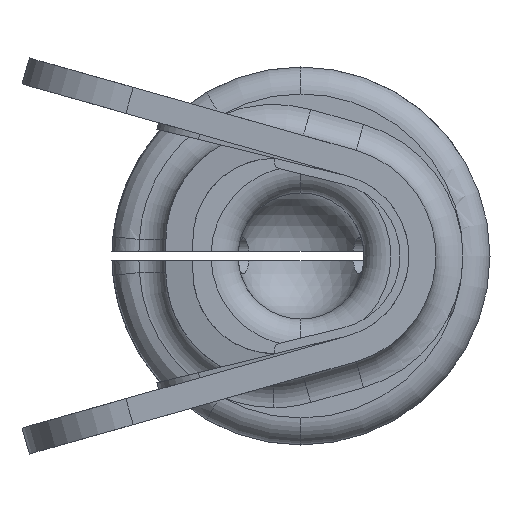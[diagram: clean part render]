
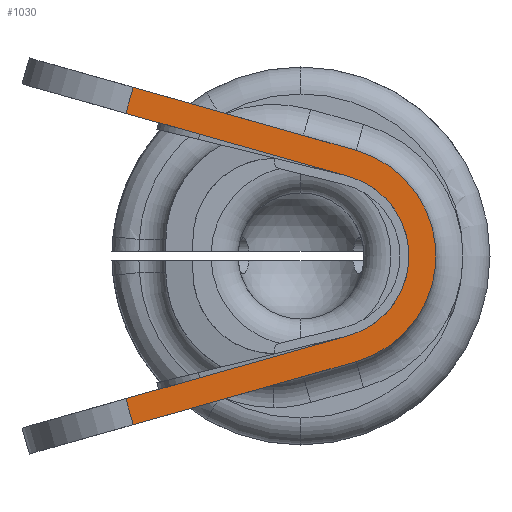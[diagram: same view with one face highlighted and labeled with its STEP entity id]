
A CAD part, left-side view. The second image highlights one B-rep face of the part: STEP entity #1030.
In plain terms, the highlighted planar face has unit normal (-1, 0, 0).
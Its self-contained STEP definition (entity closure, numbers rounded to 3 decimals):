
#196 = ORIENTED_EDGE ( 'NONE', *, *, #3248, .T. ) ;
#217 = CARTESIAN_POINT ( 'NONE',  ( -12.88, -0.106, -0.374 ) ) ;
#218 = VECTOR ( 'NONE', #5639, 1000. ) ;
#318 = ORIENTED_EDGE ( 'NONE', *, *, #1427, .T. ) ;
#349 = CIRCLE ( 'NONE', #6018, 0.46 ) ;
#354 = VECTOR ( 'NONE', #6007, 1000. ) ;
#433 = VECTOR ( 'NONE', #5708, 1000. ) ;
#526 = VERTEX_POINT ( 'NONE', #4530 ) ;
#736 = DIRECTION ( 'NONE',  ( 0., 0., -1. ) ) ;
#853 = CARTESIAN_POINT ( 'NONE',  ( -12.88, 0.26, 0. ) ) ;
#873 = EDGE_LOOP ( 'NONE', ( #5237, #196, #3596, #5016, #2593, #318, #3690, #2170 ) ) ;
#914 = VERTEX_POINT ( 'NONE', #3044 ) ;
#1030 = ADVANCED_FACE ( 'NONE', ( #2239 ), #1643, .F. ) ;
#1034 = CARTESIAN_POINT ( 'NONE',  ( -12.88, -0.147, 0.519 ) ) ;
#1427 = EDGE_CURVE ( 'NONE', #914, #5588, #1929, .T. ) ;
#1455 = CARTESIAN_POINT ( 'NONE',  ( -12.88, 1.332, -0.937 ) ) ;
#1634 = CARTESIAN_POINT ( 'NONE',  ( -12.88, 0.26, 0. ) ) ;
#1643 = PLANE ( 'NONE',  #5161 ) ;
#1670 = LINE ( 'NONE', #3774, #3249 ) ;
#1888 = CARTESIAN_POINT ( 'NONE',  ( -12.88, -0.106, 0.374 ) ) ;
#1929 = LINE ( 'NONE', #1455, #354 ) ;
#2170 = ORIENTED_EDGE ( 'NONE', *, *, #2978, .F. ) ;
#2176 = CIRCLE ( 'NONE', #4102, 0.61 ) ;
#2220 = DIRECTION ( 'NONE',  ( 0., 0.272, -0.962 ) ) ;
#2239 = FACE_OUTER_BOUND ( 'NONE', #873, .T. ) ;
#2341 = VERTEX_POINT ( 'NONE', #6127 ) ;
#2424 = DIRECTION ( 'NONE',  ( 0., -0.962, -0.272 ) ) ;
#2428 = EDGE_CURVE ( 'NONE', #5588, #526, #1670, .T. ) ;
#2438 = EDGE_CURVE ( 'NONE', #5448, #2341, #349, .T. ) ;
#2593 = ORIENTED_EDGE ( 'NONE', *, *, #5847, .F. ) ;
#2687 = CARTESIAN_POINT ( 'NONE',  ( -12.88, 0., 0. ) ) ;
#2916 = DIRECTION ( 'NONE',  ( 1., 0., 0. ) ) ;
#2974 = VERTEX_POINT ( 'NONE', #4367 ) ;
#2978 = EDGE_CURVE ( 'NONE', #6086, #526, #2176, .T. ) ;
#3028 = LINE ( 'NONE', #1034, #218 ) ;
#3044 = CARTESIAN_POINT ( 'NONE',  ( -12.88, 1.373, -0.792 ) ) ;
#3157 = DIRECTION ( 'NONE',  ( 1., 0., 0. ) ) ;
#3213 = DIRECTION ( 'NONE',  ( 0., 0., -1. ) ) ;
#3248 = EDGE_CURVE ( 'NONE', #2974, #4641, #3761, .T. ) ;
#3249 = VECTOR ( 'NONE', #5308, 1000. ) ;
#3487 = CARTESIAN_POINT ( 'NONE',  ( -12.88, 1.332, -0.937 ) ) ;
#3596 = ORIENTED_EDGE ( 'NONE', *, *, #5109, .T. ) ;
#3690 = ORIENTED_EDGE ( 'NONE', *, *, #2428, .T. ) ;
#3746 = DIRECTION ( 'NONE',  ( 1., 0., 0. ) ) ;
#3761 = LINE ( 'NONE', #6275, #6243 ) ;
#3774 = CARTESIAN_POINT ( 'NONE',  ( -12.88, -0.147, -0.519 ) ) ;
#4102 = AXIS2_PLACEMENT_3D ( 'NONE', #853, #2916, #5867 ) ;
#4283 = VECTOR ( 'NONE', #2424, 1000. ) ;
#4367 = CARTESIAN_POINT ( 'NONE',  ( -12.88, 1.332, 0.937 ) ) ;
#4530 = CARTESIAN_POINT ( 'NONE',  ( -12.88, 0.094, -0.587 ) ) ;
#4641 = VERTEX_POINT ( 'NONE', #4891 ) ;
#4891 = CARTESIAN_POINT ( 'NONE',  ( -12.88, 1.373, 0.792 ) ) ;
#4918 = LINE ( 'NONE', #1888, #4283 ) ;
#5016 = ORIENTED_EDGE ( 'NONE', *, *, #2438, .T. ) ;
#5109 = EDGE_CURVE ( 'NONE', #4641, #5448, #4918, .T. ) ;
#5130 = CARTESIAN_POINT ( 'NONE',  ( -12.88, 0.094, 0.587 ) ) ;
#5161 = AXIS2_PLACEMENT_3D ( 'NONE', #2687, #3746, #736 ) ;
#5237 = ORIENTED_EDGE ( 'NONE', *, *, #6250, .F. ) ;
#5308 = DIRECTION ( 'NONE',  ( 0., -0.962, 0.272 ) ) ;
#5337 = LINE ( 'NONE', #217, #433 ) ;
#5448 = VERTEX_POINT ( 'NONE', #5487 ) ;
#5487 = CARTESIAN_POINT ( 'NONE',  ( -12.88, 0.135, 0.442 ) ) ;
#5588 = VERTEX_POINT ( 'NONE', #3487 ) ;
#5639 = DIRECTION ( 'NONE',  ( 0., -0.962, -0.272 ) ) ;
#5708 = DIRECTION ( 'NONE',  ( 0., -0.962, 0.272 ) ) ;
#5847 = EDGE_CURVE ( 'NONE', #914, #2341, #5337, .T. ) ;
#5867 = DIRECTION ( 'NONE',  ( 0., 0., -1. ) ) ;
#6007 = DIRECTION ( 'NONE',  ( 0., -0.272, -0.962 ) ) ;
#6018 = AXIS2_PLACEMENT_3D ( 'NONE', #1634, #3157, #3213 ) ;
#6086 = VERTEX_POINT ( 'NONE', #5130 ) ;
#6127 = CARTESIAN_POINT ( 'NONE',  ( -12.88, 0.135, -0.442 ) ) ;
#6243 = VECTOR ( 'NONE', #2220, 1000. ) ;
#6250 = EDGE_CURVE ( 'NONE', #2974, #6086, #3028, .T. ) ;
#6275 = CARTESIAN_POINT ( 'NONE',  ( -12.88, 1.479, 0.418 ) ) ;
